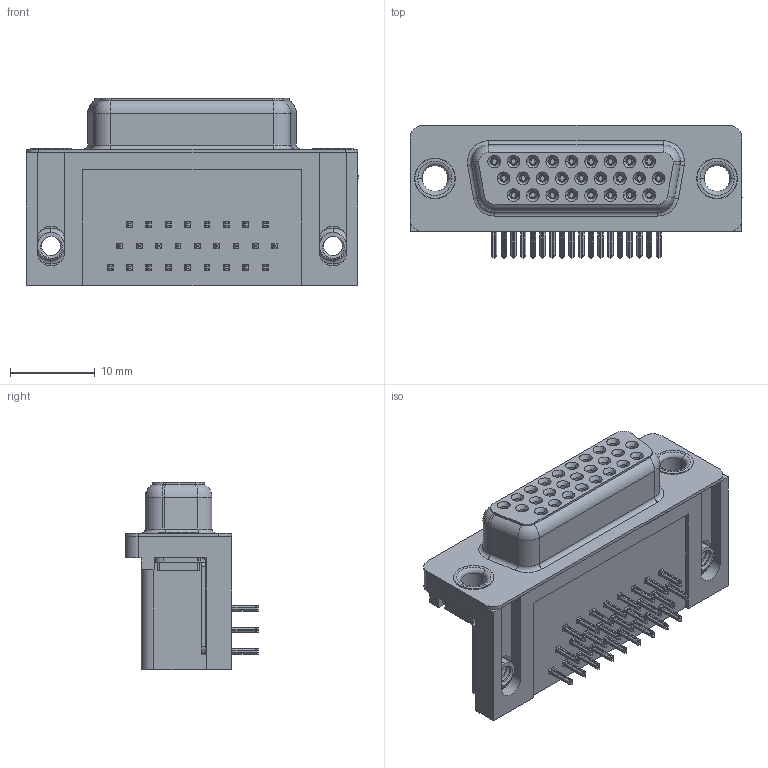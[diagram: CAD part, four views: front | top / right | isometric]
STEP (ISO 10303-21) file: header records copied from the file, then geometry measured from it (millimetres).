
FILE_DESCRIPTION (( 'STEP AP203' ), '1' );
FILE_NAME ('634-026-663-051.STEP', '2018-11-10T00:00:22', ( '' ), ( '' ), 'SwSTEP 2.0', 'SolidWorks 2016', '' );
FILE_SCHEMA (( 'CONFIG_CONTROL_DESIGN' ));
Length unit declared in the file: millimetre
Products named in the file (8): Contact Top; 4-40 Threaded Board Mount; Thru Hole Rivet; 634-026-663-051; 634 Housing_26 Socket; 634 Shell_26 Socket; Contact Bottom; Contact Middle
Assembly tree (32 placements, depth 2):
  634-026-663-051
    634 Housing_26 Socket
    634 Shell_26 Socket
    Contact Bottom  x8
    Contact Middle  x9
    Contact Top  x9
    4-40 Threaded Board Mount  x2
    Thru Hole Rivet  x2
Bounding box: 39.22 x 15.73 x 22.1 mm (x, y, z)
Volume: 6366.3 mm3; surface area: 9140.6 mm2
Topology: 32 solids, 32 shells, 3971 faces, 10434 edges, 6554 vertices
Faces by surface type: plane 1771, cylinder 932, bspline 910, cone 312, torus 46
Entity records: 36292 total; most frequent: CARTESIAN_POINT 11921, ORIENTED_EDGE 4930, DIRECTION 4372, EDGE_CURVE 2465, VERTEX_POINT 1570, VECTOR 1568, LINE 1568, AXIS2_PLACEMENT_3D 1402
